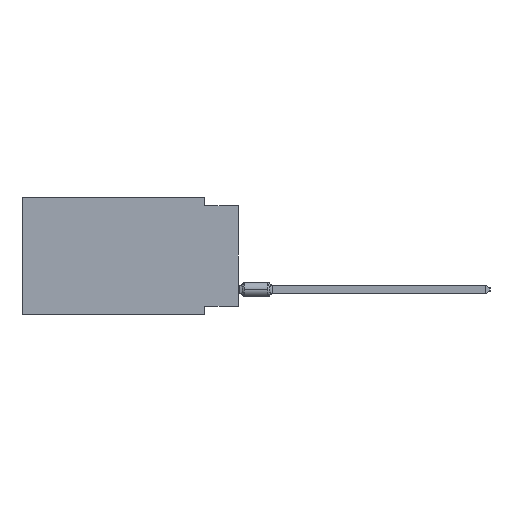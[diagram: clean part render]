
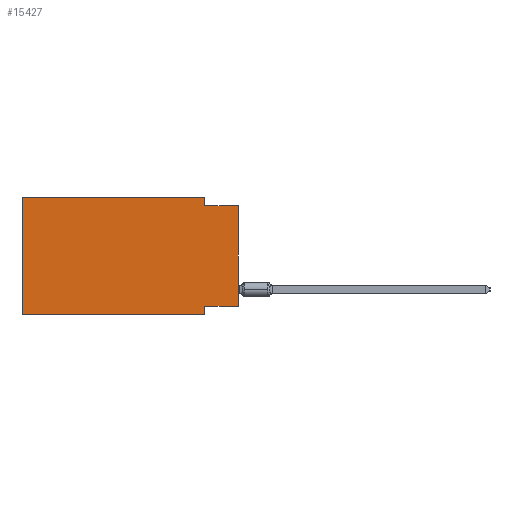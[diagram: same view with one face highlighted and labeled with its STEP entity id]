
A CAD part, left-side view. The second image highlights one B-rep face of the part: STEP entity #15427.
In plain terms, the highlighted planar face has unit normal (-1, 0, 0).
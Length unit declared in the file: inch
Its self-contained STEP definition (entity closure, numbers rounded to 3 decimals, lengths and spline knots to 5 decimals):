
#1147 = VERTEX_POINT ( 'NONE', #66535 ) ;
#1928 = EDGE_CURVE ( 'NONE', #62177, #41211, #68493, .T. ) ;
#3211 = CARTESIAN_POINT ( 'NONE',  ( 0., 0.1, 0. ) ) ;
#5362 = LINE ( 'NONE', #66475, #70235 ) ;
#9285 = FACE_OUTER_BOUND ( 'NONE', #36400, .T. ) ;
#9489 = CARTESIAN_POINT ( 'NONE',  ( 0., 0., 0. ) ) ;
#9637 = DIRECTION ( 'NONE',  ( 0., 0., -1. ) ) ;
#11005 = CARTESIAN_POINT ( 'NONE',  ( 0., 0., -0.025 ) ) ;
#11064 = VECTOR ( 'NONE', #35228, 39.37008 ) ;
#11361 = DIRECTION ( 'NONE',  ( 0., -1., 0. ) ) ;
#12845 = EDGE_CURVE ( 'NONE', #60848, #41211, #60351, .T. ) ;
#13068 = DIRECTION ( 'NONE',  ( 0., 0., 1. ) ) ;
#13786 = LINE ( 'NONE', #51312, #32261 ) ;
#13964 = DIRECTION ( 'NONE',  ( 1., 0., 0. ) ) ;
#14705 = DIRECTION ( 'NONE',  ( 0., -1., 0. ) ) ;
#14935 = EDGE_CURVE ( 'NONE', #41209, #1147, #40614, .T. ) ;
#15427 = ADVANCED_FACE ( 'NONE', ( #9285 ), #57572, .F. ) ;
#15913 = VECTOR ( 'NONE', #14705, 39.37008 ) ;
#16217 = VECTOR ( 'NONE', #9637, 39.37008 ) ;
#17501 = DIRECTION ( 'NONE',  ( 0., 1., 0. ) ) ;
#18580 = EDGE_CURVE ( 'NONE', #41209, #37484, #13786, .T. ) ;
#20032 = ORIENTED_EDGE ( 'NONE', *, *, #64731, .F. ) ;
#20802 = CARTESIAN_POINT ( 'NONE',  ( 0., 0.1, -0.35 ) ) ;
#22776 = CARTESIAN_POINT ( 'NONE',  ( 0., 0., -0.025 ) ) ;
#24530 = CARTESIAN_POINT ( 'NONE',  ( 0., 0.645, -0.35 ) ) ;
#24595 = ORIENTED_EDGE ( 'NONE', *, *, #18580, .F. ) ;
#25040 = DIRECTION ( 'NONE',  ( 0., 0., -1. ) ) ;
#25809 = CARTESIAN_POINT ( 'NONE',  ( 0., 0.1, -0.025 ) ) ;
#27202 = LINE ( 'NONE', #20802, #51620 ) ;
#30039 = CARTESIAN_POINT ( 'NONE',  ( 0., 0.645, 0. ) ) ;
#30524 = ORIENTED_EDGE ( 'NONE', *, *, #44758, .F. ) ;
#30683 = CARTESIAN_POINT ( 'NONE',  ( 0., 0.645, 0. ) ) ;
#32261 = VECTOR ( 'NONE', #13068, 39.37008 ) ;
#33126 = CARTESIAN_POINT ( 'NONE',  ( 0., 0.645, -0.35 ) ) ;
#35228 = DIRECTION ( 'NONE',  ( 0., -1., 0. ) ) ;
#36400 = EDGE_LOOP ( 'NONE', ( #41540, #57735, #56054, #30524, #24595, #37136, #20032, #43002 ) ) ;
#37136 = ORIENTED_EDGE ( 'NONE', *, *, #14935, .T. ) ;
#37208 = DIRECTION ( 'NONE',  ( 0., 0., -1. ) ) ;
#37484 = VERTEX_POINT ( 'NONE', #30683 ) ;
#40614 = LINE ( 'NONE', #24530, #11064 ) ;
#41209 = VERTEX_POINT ( 'NONE', #33126 ) ;
#41211 = VERTEX_POINT ( 'NONE', #22776 ) ;
#41540 = ORIENTED_EDGE ( 'NONE', *, *, #1928, .T. ) ;
#41857 = LINE ( 'NONE', #63674, #15913 ) ;
#42955 = VECTOR ( 'NONE', #52758, 39.37008 ) ;
#43002 = ORIENTED_EDGE ( 'NONE', *, *, #50492, .F. ) ;
#44758 = EDGE_CURVE ( 'NONE', #37484, #46349, #41857, .T. ) ;
#44915 = CARTESIAN_POINT ( 'NONE',  ( 0., 0.1, 0. ) ) ;
#46349 = VERTEX_POINT ( 'NONE', #44915 ) ;
#47883 = EDGE_CURVE ( 'NONE', #46349, #60848, #58626, .T. ) ;
#50393 = AXIS2_PLACEMENT_3D ( 'NONE', #30039, #13964, #25040 ) ;
#50492 = EDGE_CURVE ( 'NONE', #62177, #62965, #5362, .T. ) ;
#51312 = CARTESIAN_POINT ( 'NONE',  ( 0., 0.645, 0. ) ) ;
#51620 = VECTOR ( 'NONE', #37208, 39.37008 ) ;
#52758 = DIRECTION ( 'NONE',  ( 0., 0., 1. ) ) ;
#56054 = ORIENTED_EDGE ( 'NONE', *, *, #47883, .F. ) ;
#57572 = PLANE ( 'NONE',  #50393 ) ;
#57735 = ORIENTED_EDGE ( 'NONE', *, *, #12845, .F. ) ;
#58626 = LINE ( 'NONE', #3211, #16217 ) ;
#60351 = LINE ( 'NONE', #11005, #70734 ) ;
#60848 = VERTEX_POINT ( 'NONE', #25809 ) ;
#61167 = CARTESIAN_POINT ( 'NONE',  ( 0., 0., -0.325 ) ) ;
#62177 = VERTEX_POINT ( 'NONE', #61167 ) ;
#62965 = VERTEX_POINT ( 'NONE', #64273 ) ;
#63674 = CARTESIAN_POINT ( 'NONE',  ( 0., 0.645, 0. ) ) ;
#64273 = CARTESIAN_POINT ( 'NONE',  ( 0., 0.1, -0.325 ) ) ;
#64731 = EDGE_CURVE ( 'NONE', #62965, #1147, #27202, .T. ) ;
#66475 = CARTESIAN_POINT ( 'NONE',  ( 0., 0., -0.325 ) ) ;
#66535 = CARTESIAN_POINT ( 'NONE',  ( 0., 0.1, -0.35 ) ) ;
#68493 = LINE ( 'NONE', #9489, #42955 ) ;
#70235 = VECTOR ( 'NONE', #17501, 39.37008 ) ;
#70734 = VECTOR ( 'NONE', #11361, 39.37008 ) ;
